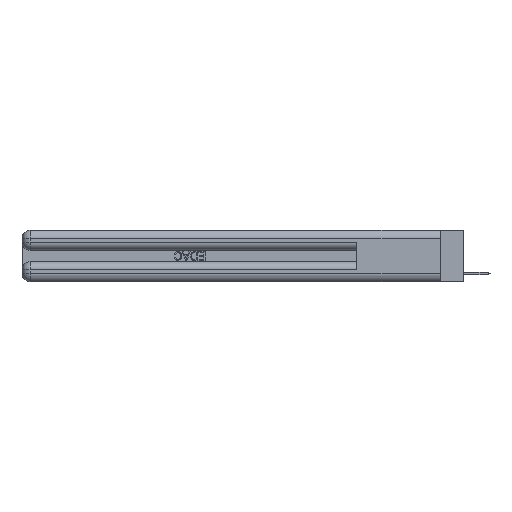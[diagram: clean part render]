
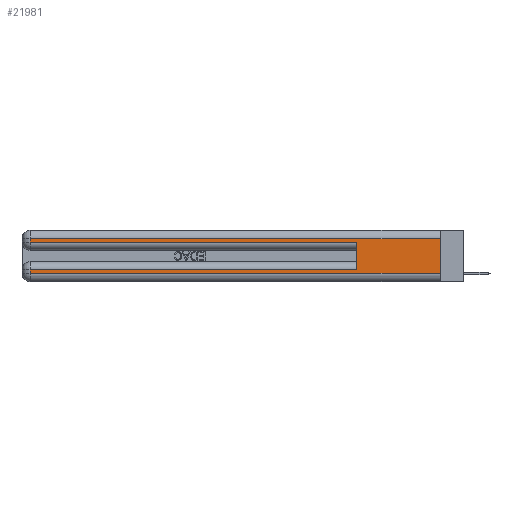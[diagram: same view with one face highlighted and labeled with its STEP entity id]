
A CAD part, left-side view. The second image highlights one B-rep face of the part: STEP entity #21981.
In plain terms, the highlighted planar face has unit normal (-1, 0, 0).
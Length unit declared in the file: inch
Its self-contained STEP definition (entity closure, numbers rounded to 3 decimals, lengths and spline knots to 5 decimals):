
#184 = VECTOR ( 'NONE', #21068, 39.37008 ) ;
#1174 = FACE_OUTER_BOUND ( 'NONE', #4896, .T. ) ;
#1259 = CARTESIAN_POINT ( 'NONE',  ( 0., 0., 0.285 ) ) ;
#1718 = LINE ( 'NONE', #21096, #5488 ) ;
#1948 = CARTESIAN_POINT ( 'NONE',  ( 0., 2.94, 0.06 ) ) ;
#2103 = ORIENTED_EDGE ( 'NONE', *, *, #5352, .F. ) ;
#2135 = CARTESIAN_POINT ( 'NONE',  ( 0., 2.94, 0.37 ) ) ;
#2410 = CARTESIAN_POINT ( 'NONE',  ( 0., 0., 0.06 ) ) ;
#3508 = DIRECTION ( 'NONE',  ( 0., 0., -1. ) ) ;
#4325 = CARTESIAN_POINT ( 'NONE',  ( 0., 2.94, 0.085 ) ) ;
#4598 = DIRECTION ( 'NONE',  ( 0., -1., 0. ) ) ;
#4896 = EDGE_LOOP ( 'NONE', ( #24534, #24266, #15665, #24755, #2103, #11656, #5238, #7488 ) ) ;
#4913 = VERTEX_POINT ( 'NONE', #1948 ) ;
#5238 = ORIENTED_EDGE ( 'NONE', *, *, #18525, .T. ) ;
#5352 = EDGE_CURVE ( 'NONE', #23757, #11435, #26099, .T. ) ;
#5488 = VECTOR ( 'NONE', #16708, 39.37008 ) ;
#7488 = ORIENTED_EDGE ( 'NONE', *, *, #9764, .T. ) ;
#7585 = VERTEX_POINT ( 'NONE', #21248 ) ;
#7642 = PLANE ( 'NONE',  #8209 ) ;
#8209 = AXIS2_PLACEMENT_3D ( 'NONE', #21015, #23201, #3508 ) ;
#8303 = CARTESIAN_POINT ( 'NONE',  ( 0., 2.94, 0.285 ) ) ;
#8345 = CARTESIAN_POINT ( 'NONE',  ( 0., 0., 0.31 ) ) ;
#8673 = DIRECTION ( 'NONE',  ( 0., 0., -1. ) ) ;
#8933 = VECTOR ( 'NONE', #25067, 39.37008 ) ;
#9160 = LINE ( 'NONE', #1259, #184 ) ;
#9696 = CARTESIAN_POINT ( 'NONE',  ( 0., 0.6, 0.145 ) ) ;
#9764 = EDGE_CURVE ( 'NONE', #4913, #11332, #18721, .T. ) ;
#11332 = VERTEX_POINT ( 'NONE', #28261 ) ;
#11435 = VERTEX_POINT ( 'NONE', #20070 ) ;
#11593 = VECTOR ( 'NONE', #11716, 39.37008 ) ;
#11656 = ORIENTED_EDGE ( 'NONE', *, *, #15803, .T. ) ;
#11716 = DIRECTION ( 'NONE',  ( 0., 0., 1. ) ) ;
#12058 = EDGE_CURVE ( 'NONE', #24002, #11332, #1718, .T. ) ;
#13737 = DIRECTION ( 'NONE',  ( 0., 1., 0. ) ) ;
#13826 = DIRECTION ( 'NONE',  ( 0., 1., 0. ) ) ;
#14166 = VECTOR ( 'NONE', #8673, 39.37008 ) ;
#14801 = LINE ( 'NONE', #18455, #8933 ) ;
#15665 = ORIENTED_EDGE ( 'NONE', *, *, #17988, .T. ) ;
#15803 = EDGE_CURVE ( 'NONE', #23757, #16664, #24319, .T. ) ;
#16664 = VERTEX_POINT ( 'NONE', #4325 ) ;
#16708 = DIRECTION ( 'NONE',  ( 0., 0., -1. ) ) ;
#16988 = VECTOR ( 'NONE', #4598, 39.37008 ) ;
#17988 = EDGE_CURVE ( 'NONE', #7585, #24213, #20038, .T. ) ;
#18455 = CARTESIAN_POINT ( 'NONE',  ( 0., 2.94, 0.37 ) ) ;
#18525 = EDGE_CURVE ( 'NONE', #16664, #4913, #14801, .T. ) ;
#18721 = LINE ( 'NONE', #2410, #16988 ) ;
#19494 = VECTOR ( 'NONE', #13737, 39.37008 ) ;
#20038 = LINE ( 'NONE', #2135, #14166 ) ;
#20070 = CARTESIAN_POINT ( 'NONE',  ( 0., 0.6, 0.285 ) ) ;
#20586 = EDGE_CURVE ( 'NONE', #24213, #11435, #9160, .T. ) ;
#20857 = VECTOR ( 'NONE', #13826, 39.37008 ) ;
#21015 = CARTESIAN_POINT ( 'NONE',  ( 0., 0., 0.37 ) ) ;
#21068 = DIRECTION ( 'NONE',  ( 0., -1., 0. ) ) ;
#21096 = CARTESIAN_POINT ( 'NONE',  ( 0., 0., 0.37 ) ) ;
#21248 = CARTESIAN_POINT ( 'NONE',  ( 0., 2.94, 0.31 ) ) ;
#21605 = LINE ( 'NONE', #22720, #19494 ) ;
#21981 = ADVANCED_FACE ( 'NONE', ( #1174 ), #7642, .F. ) ;
#22720 = CARTESIAN_POINT ( 'NONE',  ( 0., 0., 0.31 ) ) ;
#23201 = DIRECTION ( 'NONE',  ( 1., 0., 0. ) ) ;
#23757 = VERTEX_POINT ( 'NONE', #23914 ) ;
#23914 = CARTESIAN_POINT ( 'NONE',  ( 0., 0.6, 0.085 ) ) ;
#24002 = VERTEX_POINT ( 'NONE', #8345 ) ;
#24213 = VERTEX_POINT ( 'NONE', #8303 ) ;
#24266 = ORIENTED_EDGE ( 'NONE', *, *, #28341, .T. ) ;
#24319 = LINE ( 'NONE', #27077, #20857 ) ;
#24534 = ORIENTED_EDGE ( 'NONE', *, *, #12058, .F. ) ;
#24755 = ORIENTED_EDGE ( 'NONE', *, *, #20586, .T. ) ;
#25067 = DIRECTION ( 'NONE',  ( 0., 0., -1. ) ) ;
#26099 = LINE ( 'NONE', #9696, #11593 ) ;
#27077 = CARTESIAN_POINT ( 'NONE',  ( 0., 0., 0.085 ) ) ;
#28261 = CARTESIAN_POINT ( 'NONE',  ( 0., 0., 0.06 ) ) ;
#28341 = EDGE_CURVE ( 'NONE', #24002, #7585, #21605, .T. ) ;
